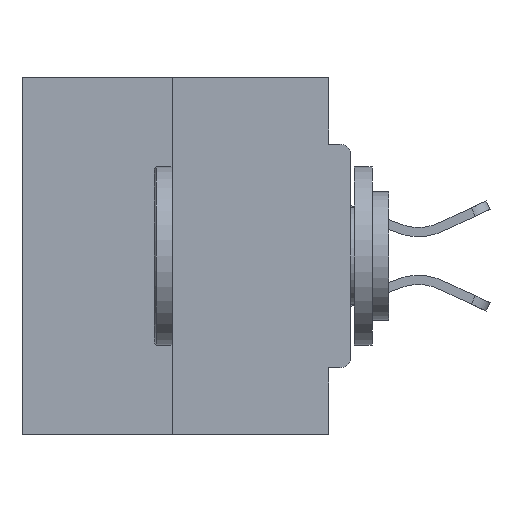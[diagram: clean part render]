
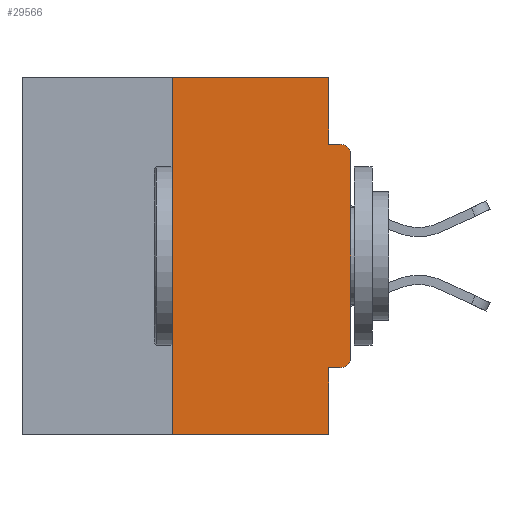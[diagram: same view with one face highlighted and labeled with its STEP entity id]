
A CAD part, left-side view. The second image highlights one B-rep face of the part: STEP entity #29566.
In plain terms, the highlighted planar face has unit normal (-1, 0, 0).
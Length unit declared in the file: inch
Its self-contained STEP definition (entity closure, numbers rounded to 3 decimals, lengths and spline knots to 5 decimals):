
#478 = DIRECTION ( 'NONE',  ( 0., 0., -1. ) ) ;
#637 = DIRECTION ( 'NONE',  ( 0., 0., -1. ) ) ;
#762 = CARTESIAN_POINT ( 'NONE',  ( 0., 0., -0.0935 ) ) ;
#849 = CARTESIAN_POINT ( 'NONE',  ( 0., 0.031, -0.0935 ) ) ;
#1145 = VERTEX_POINT ( 'NONE', #29599 ) ;
#1183 = ORIENTED_EDGE ( 'NONE', *, *, #4980, .F. ) ;
#2333 = VERTEX_POINT ( 'NONE', #5326 ) ;
#3167 = CARTESIAN_POINT ( 'NONE',  ( 0., 0.015, -0.3915 ) ) ;
#3539 = VECTOR ( 'NONE', #22890, 39.37008 ) ;
#3632 = DIRECTION ( 'NONE',  ( -1., 0., 0. ) ) ;
#4980 = EDGE_CURVE ( 'NONE', #18255, #28573, #22780, .T. ) ;
#5326 = CARTESIAN_POINT ( 'NONE',  ( 0., 0.015, -0.4065 ) ) ;
#5455 = EDGE_CURVE ( 'NONE', #5807, #1145, #22280, .T. ) ;
#5807 = VERTEX_POINT ( 'NONE', #35872 ) ;
#7055 = ORIENTED_EDGE ( 'NONE', *, *, #21621, .F. ) ;
#7227 = CARTESIAN_POINT ( 'NONE',  ( 0., 0., -0.3915 ) ) ;
#7660 = EDGE_CURVE ( 'NONE', #34494, #18255, #9874, .T. ) ;
#7706 = VECTOR ( 'NONE', #25782, 39.37008 ) ;
#8308 = AXIS2_PLACEMENT_3D ( 'NONE', #23511, #3632, #9593 ) ;
#8761 = CARTESIAN_POINT ( 'NONE',  ( 0., 0.031, 0. ) ) ;
#8908 = VECTOR ( 'NONE', #16345, 39.37008 ) ;
#9382 = EDGE_CURVE ( 'NONE', #9454, #28573, #16281, .T. ) ;
#9408 = ORIENTED_EDGE ( 'NONE', *, *, #7660, .F. ) ;
#9454 = VERTEX_POINT ( 'NONE', #23394 ) ;
#9593 = DIRECTION ( 'NONE',  ( 0., 0., -1. ) ) ;
#9874 = LINE ( 'NONE', #25662, #7706 ) ;
#10197 = EDGE_CURVE ( 'NONE', #2333, #5807, #17211, .T. ) ;
#10794 = AXIS2_PLACEMENT_3D ( 'NONE', #3167, #22707, #478 ) ;
#11294 = ORIENTED_EDGE ( 'NONE', *, *, #19932, .T. ) ;
#12214 = VECTOR ( 'NONE', #637, 39.37008 ) ;
#12263 = VECTOR ( 'NONE', #31232, 39.37008 ) ;
#13434 = CARTESIAN_POINT ( 'NONE',  ( 0., 0.46, -0.5 ) ) ;
#13525 = LINE ( 'NONE', #34452, #12263 ) ;
#14099 = CIRCLE ( 'NONE', #10794, 0.015 ) ;
#15610 = AXIS2_PLACEMENT_3D ( 'NONE', #34248, #28473, #25667 ) ;
#15819 = EDGE_CURVE ( 'NONE', #34957, #9454, #22494, .T. ) ;
#16281 = CIRCLE ( 'NONE', #8308, 0.015 ) ;
#16345 = DIRECTION ( 'NONE',  ( 0., 1., 0. ) ) ;
#16541 = ORIENTED_EDGE ( 'NONE', *, *, #15819, .T. ) ;
#17211 = LINE ( 'NONE', #27816, #8908 ) ;
#17399 = CARTESIAN_POINT ( 'NONE',  ( 0., 0.46, 0. ) ) ;
#18255 = VERTEX_POINT ( 'NONE', #849 ) ;
#18395 = LINE ( 'NONE', #17399, #3539 ) ;
#18770 = ORIENTED_EDGE ( 'NONE', *, *, #5455, .F. ) ;
#19306 = LINE ( 'NONE', #13434, #25876 ) ;
#19932 = EDGE_CURVE ( 'NONE', #2333, #34957, #14099, .T. ) ;
#20525 = CARTESIAN_POINT ( 'NONE',  ( 0., 0.015, -0.0935 ) ) ;
#20594 = EDGE_CURVE ( 'NONE', #31472, #1145, #19306, .T. ) ;
#21621 = EDGE_CURVE ( 'NONE', #30067, #34494, #18395, .T. ) ;
#22280 = LINE ( 'NONE', #23236, #12214 ) ;
#22494 = LINE ( 'NONE', #24363, #23787 ) ;
#22707 = DIRECTION ( 'NONE',  ( -1., 0., 0. ) ) ;
#22723 = FACE_OUTER_BOUND ( 'NONE', #29456, .T. ) ;
#22780 = LINE ( 'NONE', #762, #31043 ) ;
#22890 = DIRECTION ( 'NONE',  ( 0., -1., 0. ) ) ;
#22995 = DIRECTION ( 'NONE',  ( 0., -1., 0. ) ) ;
#23236 = CARTESIAN_POINT ( 'NONE',  ( 0., 0.031, -0.5 ) ) ;
#23394 = CARTESIAN_POINT ( 'NONE',  ( 0., 0., -0.1085 ) ) ;
#23511 = CARTESIAN_POINT ( 'NONE',  ( 0., 0.015, -0.1085 ) ) ;
#23746 = EDGE_CURVE ( 'NONE', #31472, #30067, #13525, .T. ) ;
#23787 = VECTOR ( 'NONE', #35720, 39.37008 ) ;
#24045 = ORIENTED_EDGE ( 'NONE', *, *, #9382, .T. ) ;
#24363 = CARTESIAN_POINT ( 'NONE',  ( 0., 0., 0. ) ) ;
#25662 = CARTESIAN_POINT ( 'NONE',  ( 0., 0.031, 0. ) ) ;
#25667 = DIRECTION ( 'NONE',  ( 0., 0., -1. ) ) ;
#25763 = ORIENTED_EDGE ( 'NONE', *, *, #10197, .F. ) ;
#25782 = DIRECTION ( 'NONE',  ( 0., 0., -1. ) ) ;
#25876 = VECTOR ( 'NONE', #30286, 39.37008 ) ;
#26614 = CARTESIAN_POINT ( 'NONE',  ( 0., 0.25, -0.5 ) ) ;
#27816 = CARTESIAN_POINT ( 'NONE',  ( 0., 0., -0.4065 ) ) ;
#28473 = DIRECTION ( 'NONE',  ( 1., 0., 0. ) ) ;
#28573 = VERTEX_POINT ( 'NONE', #20525 ) ;
#28596 = PLANE ( 'NONE',  #15610 ) ;
#29456 = EDGE_LOOP ( 'NONE', ( #7055, #35141, #35362, #18770, #25763, #11294, #16541, #24045, #1183, #9408 ) ) ;
#29566 = ADVANCED_FACE ( 'NONE', ( #22723 ), #28596, .F. ) ;
#29599 = CARTESIAN_POINT ( 'NONE',  ( 0., 0.031, -0.5 ) ) ;
#30067 = VERTEX_POINT ( 'NONE', #34029 ) ;
#30286 = DIRECTION ( 'NONE',  ( 0., -1., 0. ) ) ;
#31043 = VECTOR ( 'NONE', #22995, 39.37008 ) ;
#31232 = DIRECTION ( 'NONE',  ( 0., 0., 1. ) ) ;
#31472 = VERTEX_POINT ( 'NONE', #26614 ) ;
#34029 = CARTESIAN_POINT ( 'NONE',  ( 0., 0.25, 0. ) ) ;
#34248 = CARTESIAN_POINT ( 'NONE',  ( 0., 0.46, 0. ) ) ;
#34452 = CARTESIAN_POINT ( 'NONE',  ( 0., 0.25, 0. ) ) ;
#34494 = VERTEX_POINT ( 'NONE', #8761 ) ;
#34957 = VERTEX_POINT ( 'NONE', #7227 ) ;
#35141 = ORIENTED_EDGE ( 'NONE', *, *, #23746, .F. ) ;
#35362 = ORIENTED_EDGE ( 'NONE', *, *, #20594, .T. ) ;
#35720 = DIRECTION ( 'NONE',  ( 0., 0., 1. ) ) ;
#35872 = CARTESIAN_POINT ( 'NONE',  ( 0., 0.031, -0.4065 ) ) ;
